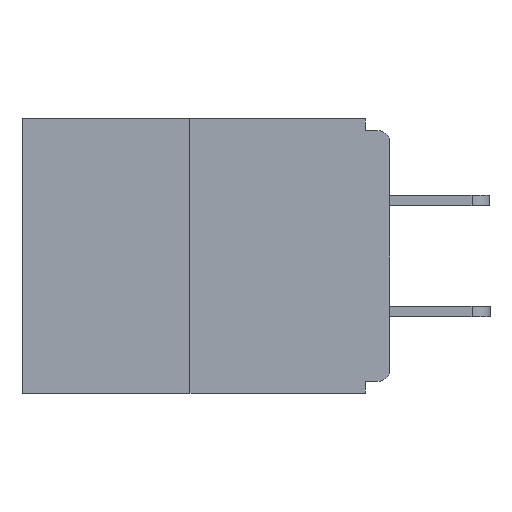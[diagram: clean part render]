
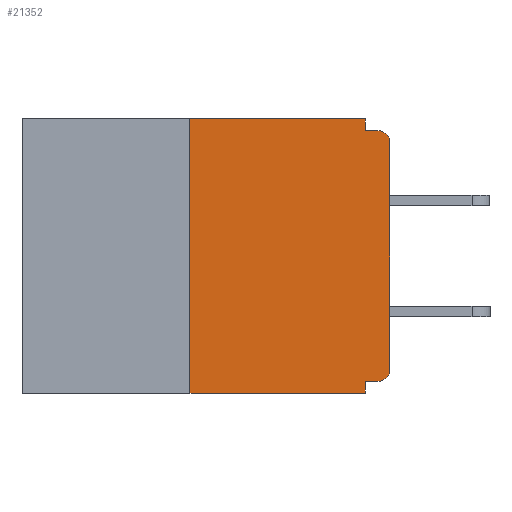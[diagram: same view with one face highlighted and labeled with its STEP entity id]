
A CAD part, left-side view. The second image highlights one B-rep face of the part: STEP entity #21352.
In plain terms, the highlighted planar face has unit normal (-1, 0, 0).
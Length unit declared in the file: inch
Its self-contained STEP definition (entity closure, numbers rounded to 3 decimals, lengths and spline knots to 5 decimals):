
#654 = CARTESIAN_POINT ( 'NONE',  ( 0., 0., -0.015 ) ) ;
#1203 = DIRECTION ( 'NONE',  ( 0., 0., 1. ) ) ;
#1998 = EDGE_CURVE ( 'NONE', #16408, #4517, #11808, .T. ) ;
#2242 = LINE ( 'NONE', #12773, #10938 ) ;
#2431 = LINE ( 'NONE', #654, #12756 ) ;
#2584 = VECTOR ( 'NONE', #18162, 39.37008 ) ;
#2677 = ORIENTED_EDGE ( 'NONE', *, *, #5679, .F. ) ;
#2781 = CARTESIAN_POINT ( 'NONE',  ( 0., 0.031, 0. ) ) ;
#2968 = EDGE_CURVE ( 'NONE', #22051, #19129, #16975, .T. ) ;
#3635 = ORIENTED_EDGE ( 'NONE', *, *, #18654, .T. ) ;
#3818 = EDGE_LOOP ( 'NONE', ( #10030, #13199, #3635, #18201, #14830, #11378, #8297, #10747, #2677, #13075 ) ) ;
#4517 = VERTEX_POINT ( 'NONE', #20888 ) ;
#4987 = VERTEX_POINT ( 'NONE', #8622 ) ;
#5679 = EDGE_CURVE ( 'NONE', #10703, #4987, #2431, .T. ) ;
#6061 = CARTESIAN_POINT ( 'NONE',  ( 0., 0.25, 0. ) ) ;
#6228 = CARTESIAN_POINT ( 'NONE',  ( 0., 0.46, 0. ) ) ;
#6433 = CARTESIAN_POINT ( 'NONE',  ( 0., 0.031, -0.343 ) ) ;
#6654 = VECTOR ( 'NONE', #21065, 39.37008 ) ;
#6943 = DIRECTION ( 'NONE',  ( 0., 0., -1. ) ) ;
#7376 = LINE ( 'NONE', #11491, #17158 ) ;
#7488 = DIRECTION ( 'NONE',  ( -1., 0., 0. ) ) ;
#7658 = LINE ( 'NONE', #13414, #20949 ) ;
#8020 = DIRECTION ( 'NONE',  ( 0., 0., -1. ) ) ;
#8297 = ORIENTED_EDGE ( 'NONE', *, *, #18233, .T. ) ;
#8622 = CARTESIAN_POINT ( 'NONE',  ( 0., 0.015, -0.015 ) ) ;
#8946 = CARTESIAN_POINT ( 'NONE',  ( 0., 0.46, 0. ) ) ;
#8995 = DIRECTION ( 'NONE',  ( -1., 0., 0. ) ) ;
#9182 = LINE ( 'NONE', #2781, #13527 ) ;
#10030 = ORIENTED_EDGE ( 'NONE', *, *, #1998, .F. ) ;
#10123 = CARTESIAN_POINT ( 'NONE',  ( 0., 0.25, 0. ) ) ;
#10703 = VERTEX_POINT ( 'NONE', #16767 ) ;
#10747 = ORIENTED_EDGE ( 'NONE', *, *, #20044, .T. ) ;
#10828 = AXIS2_PLACEMENT_3D ( 'NONE', #17902, #7488, #6943 ) ;
#10851 = EDGE_CURVE ( 'NONE', #10865, #16408, #12788, .T. ) ;
#10865 = VERTEX_POINT ( 'NONE', #11650 ) ;
#10938 = VECTOR ( 'NONE', #18120, 39.37008 ) ;
#11122 = DIRECTION ( 'NONE',  ( 0., -1., 0. ) ) ;
#11378 = ORIENTED_EDGE ( 'NONE', *, *, #12118, .T. ) ;
#11491 = CARTESIAN_POINT ( 'NONE',  ( 0., 0.46, -0.343 ) ) ;
#11650 = CARTESIAN_POINT ( 'NONE',  ( 0., 0.25, -0.343 ) ) ;
#11808 = LINE ( 'NONE', #6228, #2584 ) ;
#12118 = EDGE_CURVE ( 'NONE', #22051, #18155, #15184, .T. ) ;
#12190 = DIRECTION ( 'NONE',  ( 0., 0., -1. ) ) ;
#12247 = CARTESIAN_POINT ( 'NONE',  ( 0., 0., -0.328 ) ) ;
#12366 = EDGE_CURVE ( 'NONE', #4517, #10703, #9182, .T. ) ;
#12483 = CARTESIAN_POINT ( 'NONE',  ( 0., 0.015, -0.313 ) ) ;
#12756 = VECTOR ( 'NONE', #11122, 39.37008 ) ;
#12773 = CARTESIAN_POINT ( 'NONE',  ( 0., 0.031, -0.343 ) ) ;
#12788 = LINE ( 'NONE', #10123, #20388 ) ;
#13075 = ORIENTED_EDGE ( 'NONE', *, *, #12366, .F. ) ;
#13199 = ORIENTED_EDGE ( 'NONE', *, *, #10851, .F. ) ;
#13414 = CARTESIAN_POINT ( 'NONE',  ( 0., 0., 0. ) ) ;
#13527 = VECTOR ( 'NONE', #8020, 39.37008 ) ;
#13973 = PLANE ( 'NONE',  #20738 ) ;
#14830 = ORIENTED_EDGE ( 'NONE', *, *, #2968, .F. ) ;
#15184 = CIRCLE ( 'NONE', #22515, 0.015 ) ;
#15791 = CARTESIAN_POINT ( 'NONE',  ( 0., 0.015, -0.328 ) ) ;
#16408 = VERTEX_POINT ( 'NONE', #6061 ) ;
#16767 = CARTESIAN_POINT ( 'NONE',  ( 0., 0.031, -0.015 ) ) ;
#16975 = LINE ( 'NONE', #12247, #6654 ) ;
#17158 = VECTOR ( 'NONE', #20447, 39.37008 ) ;
#17249 = EDGE_CURVE ( 'NONE', #19129, #21932, #2242, .T. ) ;
#17487 = DIRECTION ( 'NONE',  ( 1., 0., 0. ) ) ;
#17902 = CARTESIAN_POINT ( 'NONE',  ( 0., 0.015, -0.03 ) ) ;
#18093 = CARTESIAN_POINT ( 'NONE',  ( 0., 0., -0.03 ) ) ;
#18120 = DIRECTION ( 'NONE',  ( 0., 0., -1. ) ) ;
#18155 = VERTEX_POINT ( 'NONE', #20115 ) ;
#18162 = DIRECTION ( 'NONE',  ( 0., -1., 0. ) ) ;
#18201 = ORIENTED_EDGE ( 'NONE', *, *, #17249, .F. ) ;
#18233 = EDGE_CURVE ( 'NONE', #18155, #18886, #7658, .T. ) ;
#18654 = EDGE_CURVE ( 'NONE', #10865, #21932, #7376, .T. ) ;
#18886 = VERTEX_POINT ( 'NONE', #18093 ) ;
#19129 = VERTEX_POINT ( 'NONE', #19642 ) ;
#19594 = FACE_OUTER_BOUND ( 'NONE', #3818, .T. ) ;
#19642 = CARTESIAN_POINT ( 'NONE',  ( 0., 0.031, -0.328 ) ) ;
#20044 = EDGE_CURVE ( 'NONE', #18886, #4987, #22054, .T. ) ;
#20115 = CARTESIAN_POINT ( 'NONE',  ( 0., 0., -0.313 ) ) ;
#20388 = VECTOR ( 'NONE', #20623, 39.37008 ) ;
#20447 = DIRECTION ( 'NONE',  ( 0., -1., 0. ) ) ;
#20623 = DIRECTION ( 'NONE',  ( 0., 0., 1. ) ) ;
#20738 = AXIS2_PLACEMENT_3D ( 'NONE', #8946, #17487, #21195 ) ;
#20888 = CARTESIAN_POINT ( 'NONE',  ( 0., 0.031, 0. ) ) ;
#20949 = VECTOR ( 'NONE', #1203, 39.37008 ) ;
#21065 = DIRECTION ( 'NONE',  ( 0., 1., 0. ) ) ;
#21195 = DIRECTION ( 'NONE',  ( 0., 0., -1. ) ) ;
#21352 = ADVANCED_FACE ( 'NONE', ( #19594 ), #13973, .F. ) ;
#21932 = VERTEX_POINT ( 'NONE', #6433 ) ;
#22051 = VERTEX_POINT ( 'NONE', #15791 ) ;
#22054 = CIRCLE ( 'NONE', #10828, 0.015 ) ;
#22515 = AXIS2_PLACEMENT_3D ( 'NONE', #12483, #8995, #12190 ) ;
